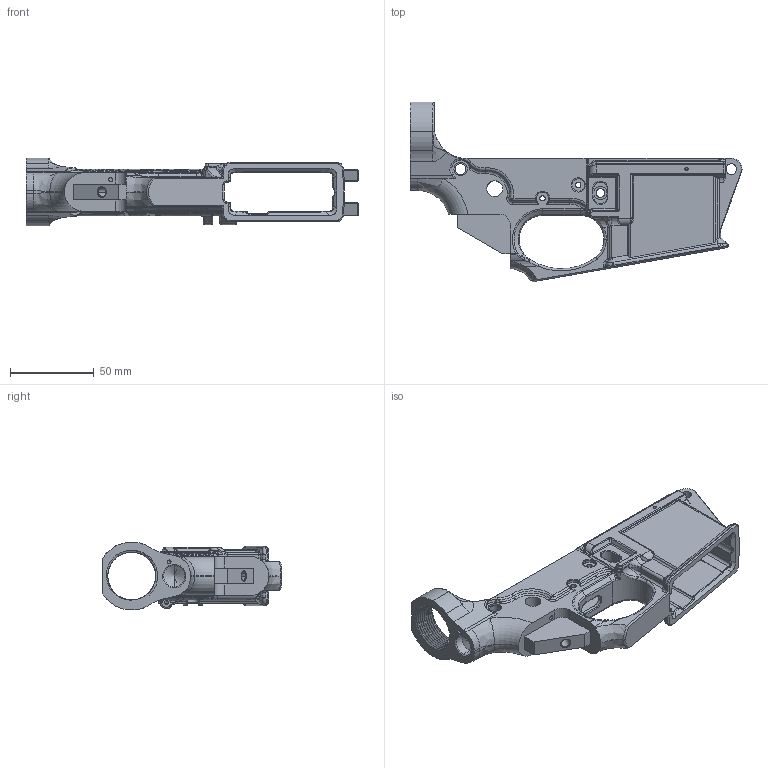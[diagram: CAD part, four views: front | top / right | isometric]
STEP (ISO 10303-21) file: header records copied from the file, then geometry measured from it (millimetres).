
FILE_DESCRIPTION (( 'STEP AP203' ), '1' );
FILE_NAME ('CW-3DPrint-AR15-Lower.STEP', '2021-02-20T22:56:54', ( '' ), ( '' ), 'SwSTEP 2.0', 'SolidWorks 2020', '' );
FILE_SCHEMA (( 'CONFIG_CONTROL_DESIGN' ));
Products named in the file (1): CW-3DPrint-AR15-Lower
Bounding box: 198.51 x 107.48 x 40.6 mm (x, y, z)
Surface area: 56671.2 mm2 (no closed solid volume)
Topology: 0 solids, 2 shells, 1229 faces, 3171 edges, 1925 vertices
Faces by surface type: bspline 400, cylinder 386, plane 272, torus 117, cone 36, sphere 18
Entity records: 73188 total; most frequent: CARTESIAN_POINT 46755, ORIENTED_EDGE 6262, DIRECTION 4495, EDGE_CURVE 3133, VERTEX_POINT 1923, AXIS2_PLACEMENT_3D 1640, EDGE_LOOP 1289, FACE_OUTER_BOUND 1229
